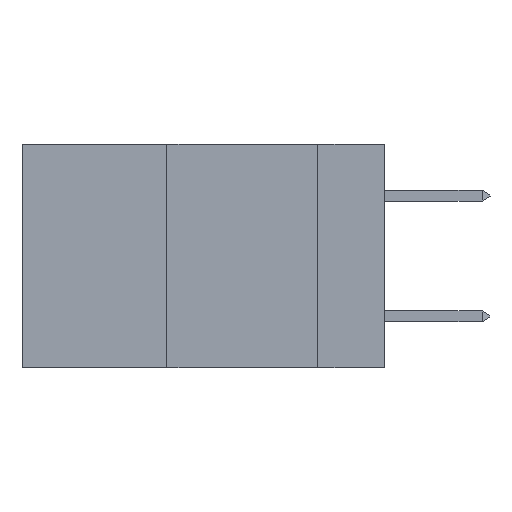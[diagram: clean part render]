
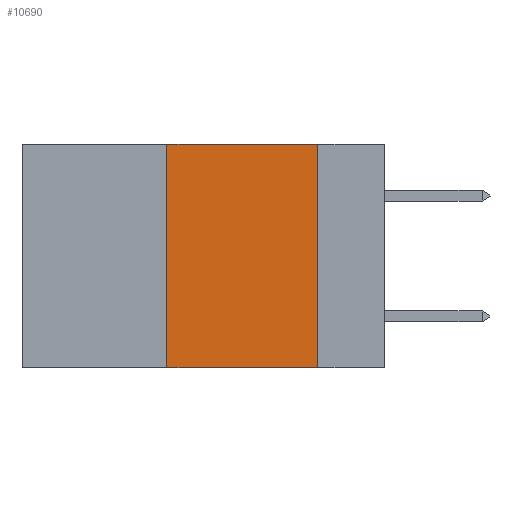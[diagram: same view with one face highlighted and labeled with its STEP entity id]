
A CAD part, left-side view. The second image highlights one B-rep face of the part: STEP entity #10690.
In plain terms, the highlighted planar face has unit normal (-1, 0, 0).
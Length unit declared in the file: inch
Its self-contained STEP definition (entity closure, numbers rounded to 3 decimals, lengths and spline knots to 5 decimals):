
#90 = PLANE ( 'NONE',  #5424 ) ;
#1092 = VECTOR ( 'NONE', #7982, 39.37008 ) ;
#1598 = CARTESIAN_POINT ( 'NONE',  ( 0., 0.6, 0. ) ) ;
#2203 = DIRECTION ( 'NONE',  ( 0., 0., 1. ) ) ;
#2206 = EDGE_CURVE ( 'NONE', #2598, #5025, #10125, .T. ) ;
#2269 = CARTESIAN_POINT ( 'NONE',  ( 0., 0.36, 0. ) ) ;
#2598 = VERTEX_POINT ( 'NONE', #4338 ) ;
#3986 = CARTESIAN_POINT ( 'NONE',  ( 0., 0.36, -0.37 ) ) ;
#3992 = CARTESIAN_POINT ( 'NONE',  ( 0., 0.6, -0.37 ) ) ;
#4029 = CARTESIAN_POINT ( 'NONE',  ( 0., 0.11, 0. ) ) ;
#4044 = VECTOR ( 'NONE', #11275, 39.37008 ) ;
#4127 = VERTEX_POINT ( 'NONE', #3986 ) ;
#4173 = ORIENTED_EDGE ( 'NONE', *, *, #6165, .T. ) ;
#4338 = CARTESIAN_POINT ( 'NONE',  ( 0., 0.11, 0. ) ) ;
#5025 = VERTEX_POINT ( 'NONE', #8765 ) ;
#5161 = EDGE_LOOP ( 'NONE', ( #9121, #5748, #5551, #4173 ) ) ;
#5424 = AXIS2_PLACEMENT_3D ( 'NONE', #7117, #12106, #12708 ) ;
#5491 = VECTOR ( 'NONE', #2203, 39.37008 ) ;
#5551 = ORIENTED_EDGE ( 'NONE', *, *, #5695, .F. ) ;
#5695 = EDGE_CURVE ( 'NONE', #4127, #6533, #7200, .T. ) ;
#5748 = ORIENTED_EDGE ( 'NONE', *, *, #5849, .F. ) ;
#5849 = EDGE_CURVE ( 'NONE', #6533, #2598, #10498, .T. ) ;
#6165 = EDGE_CURVE ( 'NONE', #4127, #5025, #6202, .T. ) ;
#6202 = LINE ( 'NONE', #3992, #8813 ) ;
#6533 = VERTEX_POINT ( 'NONE', #9022 ) ;
#7117 = CARTESIAN_POINT ( 'NONE',  ( 0., 0.6, 0. ) ) ;
#7190 = FACE_OUTER_BOUND ( 'NONE', #5161, .T. ) ;
#7200 = LINE ( 'NONE', #2269, #5491 ) ;
#7946 = DIRECTION ( 'NONE',  ( 0., -1., 0. ) ) ;
#7982 = DIRECTION ( 'NONE',  ( 0., 0., -1. ) ) ;
#8765 = CARTESIAN_POINT ( 'NONE',  ( 0., 0.11, -0.37 ) ) ;
#8813 = VECTOR ( 'NONE', #7946, 39.37008 ) ;
#9022 = CARTESIAN_POINT ( 'NONE',  ( 0., 0.36, 0. ) ) ;
#9121 = ORIENTED_EDGE ( 'NONE', *, *, #2206, .F. ) ;
#10125 = LINE ( 'NONE', #4029, #1092 ) ;
#10498 = LINE ( 'NONE', #1598, #4044 ) ;
#10690 = ADVANCED_FACE ( 'NONE', ( #7190 ), #90, .F. ) ;
#11275 = DIRECTION ( 'NONE',  ( 0., -1., 0. ) ) ;
#12106 = DIRECTION ( 'NONE',  ( 1., 0., 0. ) ) ;
#12708 = DIRECTION ( 'NONE',  ( 0., 0., -1. ) ) ;
